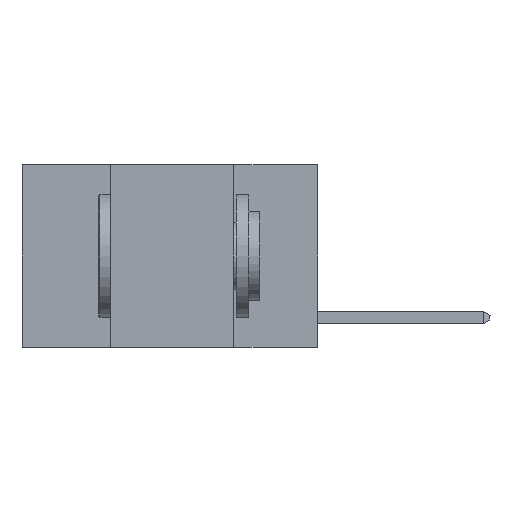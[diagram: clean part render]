
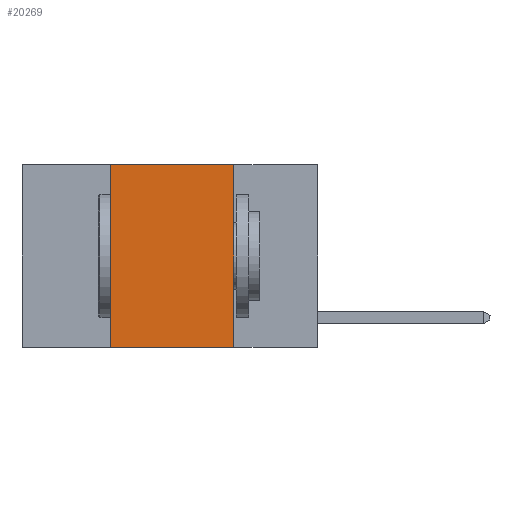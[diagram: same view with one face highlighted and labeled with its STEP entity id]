
A CAD part, left-side view. The second image highlights one B-rep face of the part: STEP entity #20269.
In plain terms, the highlighted planar face has unit normal (-1, 0, 0).
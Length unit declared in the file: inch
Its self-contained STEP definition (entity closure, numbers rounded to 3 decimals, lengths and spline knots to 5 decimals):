
#934 = VERTEX_POINT ( 'NONE', #23729 ) ;
#2333 = DIRECTION ( 'NONE',  ( 0., 0., -1. ) ) ;
#2974 = CARTESIAN_POINT ( 'NONE',  ( 0., 0.17, 0. ) ) ;
#4628 = VERTEX_POINT ( 'NONE', #2974 ) ;
#4635 = CARTESIAN_POINT ( 'NONE',  ( 0., 0.6, 0. ) ) ;
#5273 = CARTESIAN_POINT ( 'NONE',  ( 0., 0.42, 0. ) ) ;
#5788 = FACE_OUTER_BOUND ( 'NONE', #12524, .T. ) ;
#5789 = AXIS2_PLACEMENT_3D ( 'NONE', #4635, #17530, #6499 ) ;
#6499 = DIRECTION ( 'NONE',  ( 0., 0., -1. ) ) ;
#6872 = CARTESIAN_POINT ( 'NONE',  ( 0., 0.6, 0. ) ) ;
#7274 = LINE ( 'NONE', #22603, #11012 ) ;
#7472 = LINE ( 'NONE', #6872, #20421 ) ;
#7718 = VECTOR ( 'NONE', #19034, 39.37008 ) ;
#8017 = CARTESIAN_POINT ( 'NONE',  ( 0., 0.6, -0.37 ) ) ;
#8196 = LINE ( 'NONE', #5273, #22310 ) ;
#10542 = EDGE_CURVE ( 'NONE', #4628, #22015, #7274, .T. ) ;
#11012 = VECTOR ( 'NONE', #2333, 39.37008 ) ;
#11306 = CARTESIAN_POINT ( 'NONE',  ( 0., 0.42, 0. ) ) ;
#12208 = VERTEX_POINT ( 'NONE', #11306 ) ;
#12485 = EDGE_CURVE ( 'NONE', #12208, #4628, #7472, .T. ) ;
#12524 = EDGE_LOOP ( 'NONE', ( #15216, #21292, #16952, #12623 ) ) ;
#12623 = ORIENTED_EDGE ( 'NONE', *, *, #14194, .T. ) ;
#14194 = EDGE_CURVE ( 'NONE', #934, #22015, #17495, .T. ) ;
#14530 = DIRECTION ( 'NONE',  ( 0., 0., 1. ) ) ;
#15216 = ORIENTED_EDGE ( 'NONE', *, *, #10542, .F. ) ;
#16952 = ORIENTED_EDGE ( 'NONE', *, *, #22886, .F. ) ;
#17495 = LINE ( 'NONE', #8017, #7718 ) ;
#17530 = DIRECTION ( 'NONE',  ( 1., 0., 0. ) ) ;
#19034 = DIRECTION ( 'NONE',  ( 0., -1., 0. ) ) ;
#20269 = ADVANCED_FACE ( 'NONE', ( #5788 ), #21162, .F. ) ;
#20421 = VECTOR ( 'NONE', #21624, 39.37008 ) ;
#20867 = CARTESIAN_POINT ( 'NONE',  ( 0., 0.17, -0.37 ) ) ;
#21162 = PLANE ( 'NONE',  #5789 ) ;
#21292 = ORIENTED_EDGE ( 'NONE', *, *, #12485, .F. ) ;
#21624 = DIRECTION ( 'NONE',  ( 0., -1., 0. ) ) ;
#22015 = VERTEX_POINT ( 'NONE', #20867 ) ;
#22310 = VECTOR ( 'NONE', #14530, 39.37008 ) ;
#22603 = CARTESIAN_POINT ( 'NONE',  ( 0., 0.17, 0. ) ) ;
#22886 = EDGE_CURVE ( 'NONE', #934, #12208, #8196, .T. ) ;
#23729 = CARTESIAN_POINT ( 'NONE',  ( 0., 0.42, -0.37 ) ) ;
